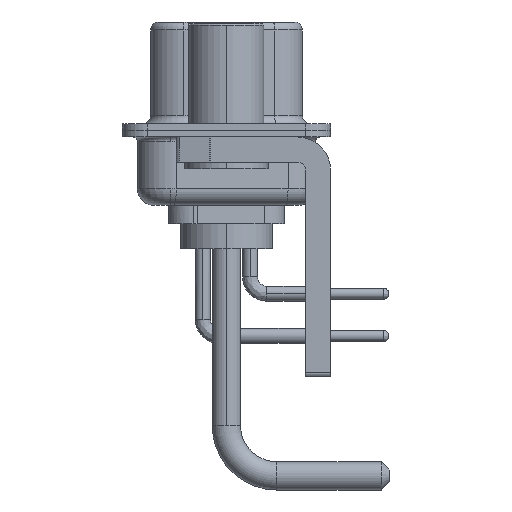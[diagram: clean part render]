
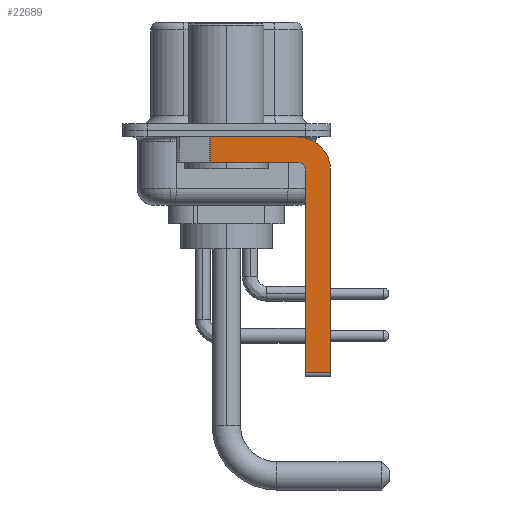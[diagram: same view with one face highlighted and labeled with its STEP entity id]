
A CAD part, left-side view. The second image highlights one B-rep face of the part: STEP entity #22689.
In plain terms, the highlighted planar face has unit normal (-1, 0, 0).
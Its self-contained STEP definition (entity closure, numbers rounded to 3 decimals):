
#116 = CARTESIAN_POINT ( 'NONE',  ( -2.9, -4.75, -2.4 ) ) ;
#197 = CARTESIAN_POINT ( 'NONE',  ( -2.9, -4.25, -0.4 ) ) ;
#242 = LINE ( 'NONE', #3561, #16836 ) ;
#435 = DIRECTION ( 'NONE',  ( 0., 0., -1. ) ) ;
#458 = LINE ( 'NONE', #13017, #8447 ) ;
#743 = ORIENTED_EDGE ( 'NONE', *, *, #6220, .T. ) ;
#1308 = CARTESIAN_POINT ( 'NONE',  ( -2.9, -4.25, -1.9 ) ) ;
#1462 = EDGE_CURVE ( 'NONE', #11440, #14805, #13609, .T. ) ;
#1710 = VERTEX_POINT ( 'NONE', #23306 ) ;
#2018 = CARTESIAN_POINT ( 'NONE',  ( -2.9, -4.25, -2.4 ) ) ;
#2101 = DIRECTION ( 'NONE',  ( 0., 0., -1. ) ) ;
#2634 = AXIS2_PLACEMENT_3D ( 'NONE', #2018, #6106, #10352 ) ;
#3237 = DIRECTION ( 'NONE',  ( 0., 1., 0. ) ) ;
#3561 = CARTESIAN_POINT ( 'NONE',  ( -2.9, -4.75, -14.8 ) ) ;
#3932 = DIRECTION ( 'NONE',  ( 0., 0., -1. ) ) ;
#4244 = AXIS2_PLACEMENT_3D ( 'NONE', #19151, #6981, #435 ) ;
#5397 = EDGE_CURVE ( 'NONE', #1710, #25543, #10429, .T. ) ;
#5645 = DIRECTION ( 'NONE',  ( 0., -1., 0. ) ) ;
#6106 = DIRECTION ( 'NONE',  ( -1., 0., 0. ) ) ;
#6220 = EDGE_CURVE ( 'NONE', #9900, #14805, #7746, .T. ) ;
#6472 = CARTESIAN_POINT ( 'NONE',  ( -2.9, -6.25, -2.4 ) ) ;
#6825 = ORIENTED_EDGE ( 'NONE', *, *, #18660, .F. ) ;
#6981 = DIRECTION ( 'NONE',  ( 1., 0., 0. ) ) ;
#7093 = VECTOR ( 'NONE', #5645, 1000. ) ;
#7659 = EDGE_CURVE ( 'NONE', #10184, #11440, #22712, .T. ) ;
#7663 = EDGE_LOOP ( 'NONE', ( #9613, #743, #11341, #17532, #6825, #24247, #12834, #25331 ) ) ;
#7746 = LINE ( 'NONE', #22646, #13068 ) ;
#8447 = VECTOR ( 'NONE', #20957, 1000. ) ;
#8602 = CARTESIAN_POINT ( 'NONE',  ( -2.9, -4.75, -14.55 ) ) ;
#8886 = CARTESIAN_POINT ( 'NONE',  ( -2.9, 0.978, -0.4 ) ) ;
#9613 = ORIENTED_EDGE ( 'NONE', *, *, #15205, .F. ) ;
#9900 = VERTEX_POINT ( 'NONE', #8886 ) ;
#10184 = VERTEX_POINT ( 'NONE', #116 ) ;
#10209 = AXIS2_PLACEMENT_3D ( 'NONE', #26103, #22145, #15724 ) ;
#10227 = VECTOR ( 'NONE', #2101, 1000. ) ;
#10352 = DIRECTION ( 'NONE',  ( 0., 0., 1. ) ) ;
#10429 = LINE ( 'NONE', #6472, #10227 ) ;
#10945 = FACE_OUTER_BOUND ( 'NONE', #7663, .T. ) ;
#11341 = ORIENTED_EDGE ( 'NONE', *, *, #1462, .F. ) ;
#11440 = VERTEX_POINT ( 'NONE', #16639 ) ;
#12603 = EDGE_CURVE ( 'NONE', #23773, #1710, #25478, .T. ) ;
#12657 = DIRECTION ( 'NONE',  ( 0., 0., 1. ) ) ;
#12834 = ORIENTED_EDGE ( 'NONE', *, *, #5397, .F. ) ;
#13017 = CARTESIAN_POINT ( 'NONE',  ( -2.9, -4.25, -14.55 ) ) ;
#13068 = VECTOR ( 'NONE', #3932, 1000. ) ;
#13609 = LINE ( 'NONE', #1308, #16254 ) ;
#14378 = CARTESIAN_POINT ( 'NONE',  ( -2.9, 3., -0.4 ) ) ;
#14805 = VERTEX_POINT ( 'NONE', #15974 ) ;
#15205 = EDGE_CURVE ( 'NONE', #9900, #23773, #16429, .T. ) ;
#15724 = DIRECTION ( 'NONE',  ( 0., 0., -1. ) ) ;
#15735 = VERTEX_POINT ( 'NONE', #8602 ) ;
#15974 = CARTESIAN_POINT ( 'NONE',  ( -2.9, 0.978, -1.9 ) ) ;
#16254 = VECTOR ( 'NONE', #3237, 1000. ) ;
#16429 = LINE ( 'NONE', #14378, #7093 ) ;
#16504 = EDGE_CURVE ( 'NONE', #15735, #25543, #458, .T. ) ;
#16639 = CARTESIAN_POINT ( 'NONE',  ( -2.9, -4.25, -1.9 ) ) ;
#16836 = VECTOR ( 'NONE', #12657, 1000. ) ;
#17532 = ORIENTED_EDGE ( 'NONE', *, *, #7659, .F. ) ;
#18660 = EDGE_CURVE ( 'NONE', #15735, #10184, #242, .T. ) ;
#19151 = CARTESIAN_POINT ( 'NONE',  ( -2.9, -4.25, -2.4 ) ) ;
#19684 = PLANE ( 'NONE',  #4244 ) ;
#20957 = DIRECTION ( 'NONE',  ( 0., -1., 0. ) ) ;
#22145 = DIRECTION ( 'NONE',  ( 1., 0., 0. ) ) ;
#22646 = CARTESIAN_POINT ( 'NONE',  ( -2.9, 0.978, -1.9 ) ) ;
#22689 = ADVANCED_FACE ( 'NONE', ( #10945 ), #19684, .F. ) ;
#22712 = CIRCLE ( 'NONE', #2634, 0.5 ) ;
#23306 = CARTESIAN_POINT ( 'NONE',  ( -2.9, -6.25, -2.4 ) ) ;
#23773 = VERTEX_POINT ( 'NONE', #197 ) ;
#24247 = ORIENTED_EDGE ( 'NONE', *, *, #16504, .T. ) ;
#24763 = CARTESIAN_POINT ( 'NONE',  ( -2.9, -6.25, -14.55 ) ) ;
#25331 = ORIENTED_EDGE ( 'NONE', *, *, #12603, .F. ) ;
#25478 = CIRCLE ( 'NONE', #10209, 2. ) ;
#25543 = VERTEX_POINT ( 'NONE', #24763 ) ;
#26103 = CARTESIAN_POINT ( 'NONE',  ( -2.9, -4.25, -2.4 ) ) ;
